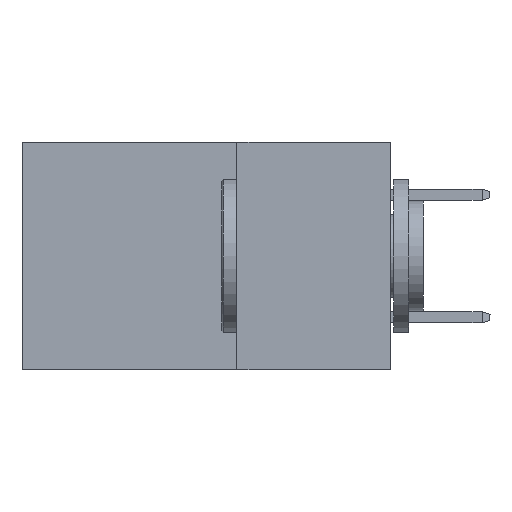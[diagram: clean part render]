
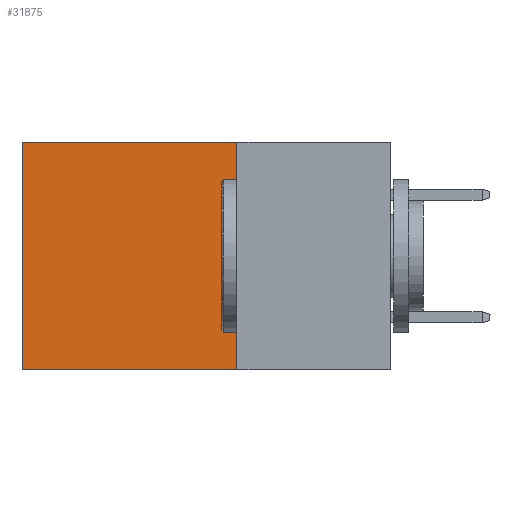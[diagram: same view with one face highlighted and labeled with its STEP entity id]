
A CAD part, left-side view. The second image highlights one B-rep face of the part: STEP entity #31875.
In plain terms, the highlighted planar face has unit normal (-1, 0, 0).
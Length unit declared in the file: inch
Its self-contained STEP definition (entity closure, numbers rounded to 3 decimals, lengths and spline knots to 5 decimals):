
#1377 = CARTESIAN_POINT ( 'NONE',  ( 0.2875, 0.6, -0.37 ) ) ;
#2647 = LINE ( 'NONE', #19002, #10516 ) ;
#3178 = CARTESIAN_POINT ( 'NONE',  ( 0.2875, 0.25, 0. ) ) ;
#3880 = LINE ( 'NONE', #22659, #35967 ) ;
#4438 = ORIENTED_EDGE ( 'NONE', *, *, #28148, .T. ) ;
#4958 = VERTEX_POINT ( 'NONE', #19249 ) ;
#5120 = CARTESIAN_POINT ( 'NONE',  ( 0.2875, 0.25, -0.37 ) ) ;
#8015 = DIRECTION ( 'NONE',  ( 0., 1., 0. ) ) ;
#9055 = ORIENTED_EDGE ( 'NONE', *, *, #40812, .F. ) ;
#9502 = CARTESIAN_POINT ( 'NONE',  ( 0.2875, 0.25, -0.37 ) ) ;
#10516 = VECTOR ( 'NONE', #19144, 39.37008 ) ;
#10596 = CARTESIAN_POINT ( 'NONE',  ( 0.2875, 0.25, 0. ) ) ;
#11655 = FACE_OUTER_BOUND ( 'NONE', #21368, .T. ) ;
#12292 = LINE ( 'NONE', #5120, #29589 ) ;
#12607 = LINE ( 'NONE', #3178, #24947 ) ;
#13398 = VERTEX_POINT ( 'NONE', #19424 ) ;
#13694 = VERTEX_POINT ( 'NONE', #1377 ) ;
#13876 = ORIENTED_EDGE ( 'NONE', *, *, #38125, .F. ) ;
#15970 = PLANE ( 'NONE',  #39858 ) ;
#15981 = EDGE_CURVE ( 'NONE', #4958, #13398, #12607, .T. ) ;
#19002 = CARTESIAN_POINT ( 'NONE',  ( 0.2875, 0.6, 0. ) ) ;
#19144 = DIRECTION ( 'NONE',  ( 0., 0., -1. ) ) ;
#19249 = CARTESIAN_POINT ( 'NONE',  ( 0.2875, 0.25, 0. ) ) ;
#19424 = CARTESIAN_POINT ( 'NONE',  ( 0.2875, 0.6, 0. ) ) ;
#20639 = VERTEX_POINT ( 'NONE', #9502 ) ;
#21368 = EDGE_LOOP ( 'NONE', ( #4438, #13876, #9055, #39122 ) ) ;
#22659 = CARTESIAN_POINT ( 'NONE',  ( 0.2875, 0.25, 0. ) ) ;
#22748 = DIRECTION ( 'NONE',  ( 0., 0., -1. ) ) ;
#24947 = VECTOR ( 'NONE', #31459, 39.37008 ) ;
#25270 = DIRECTION ( 'NONE',  ( 0., 0., -1. ) ) ;
#26182 = DIRECTION ( 'NONE',  ( 1., 0., 0. ) ) ;
#28148 = EDGE_CURVE ( 'NONE', #13398, #13694, #2647, .T. ) ;
#29589 = VECTOR ( 'NONE', #8015, 39.37008 ) ;
#31459 = DIRECTION ( 'NONE',  ( 0., 1., 0. ) ) ;
#31875 = ADVANCED_FACE ( 'NONE', ( #11655 ), #15970, .F. ) ;
#35967 = VECTOR ( 'NONE', #25270, 39.37008 ) ;
#38125 = EDGE_CURVE ( 'NONE', #20639, #13694, #12292, .T. ) ;
#39122 = ORIENTED_EDGE ( 'NONE', *, *, #15981, .T. ) ;
#39858 = AXIS2_PLACEMENT_3D ( 'NONE', #10596, #26182, #22748 ) ;
#40812 = EDGE_CURVE ( 'NONE', #4958, #20639, #3880, .T. ) ;
